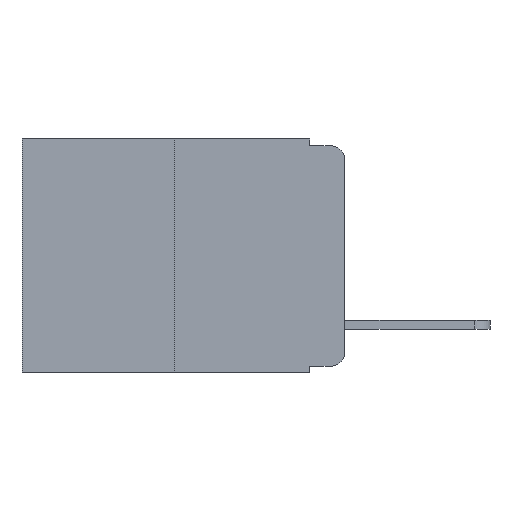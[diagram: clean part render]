
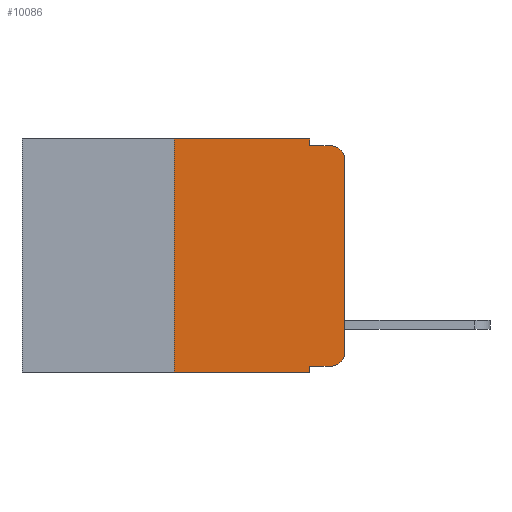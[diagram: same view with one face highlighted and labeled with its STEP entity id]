
A CAD part, left-side view. The second image highlights one B-rep face of the part: STEP entity #10086.
In plain terms, the highlighted planar face has unit normal (-1, 0, 0).
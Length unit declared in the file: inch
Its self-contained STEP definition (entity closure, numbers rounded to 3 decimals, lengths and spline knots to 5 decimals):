
#522 = VERTEX_POINT ( 'NONE', #17856 ) ;
#635 = EDGE_LOOP ( 'NONE', ( #8766, #15055, #14808, #16039, #1866, #13015, #6742, #17169, #10943, #3897 ) ) ;
#1286 = VERTEX_POINT ( 'NONE', #6475 ) ;
#1456 = CARTESIAN_POINT ( 'NONE',  ( 0., 0.473, 0. ) ) ;
#1482 = VECTOR ( 'NONE', #19501, 39.37008 ) ;
#1515 = VERTEX_POINT ( 'NONE', #21217 ) ;
#1670 = VERTEX_POINT ( 'NONE', #19282 ) ;
#1773 = VERTEX_POINT ( 'NONE', #13369 ) ;
#1866 = ORIENTED_EDGE ( 'NONE', *, *, #22059, .F. ) ;
#2009 = CARTESIAN_POINT ( 'NONE',  ( 0., 0.051, 0. ) ) ;
#2374 = DIRECTION ( 'NONE',  ( 0., -1., 0. ) ) ;
#2985 = DIRECTION ( 'NONE',  ( 1., 0., 0. ) ) ;
#3339 = LINE ( 'NONE', #13396, #12637 ) ;
#3429 = CARTESIAN_POINT ( 'NONE',  ( 0., 0.25, 0. ) ) ;
#3896 = CARTESIAN_POINT ( 'NONE',  ( 0., 0.02, -0.03 ) ) ;
#3897 = ORIENTED_EDGE ( 'NONE', *, *, #13821, .T. ) ;
#4134 = CARTESIAN_POINT ( 'NONE',  ( 0., 0., 0. ) ) ;
#4506 = LINE ( 'NONE', #16288, #18839 ) ;
#4828 = DIRECTION ( 'NONE',  ( -1., 0., 0. ) ) ;
#5191 = FACE_OUTER_BOUND ( 'NONE', #635, .T. ) ;
#5211 = AXIS2_PLACEMENT_3D ( 'NONE', #15558, #4828, #17143 ) ;
#5690 = DIRECTION ( 'NONE',  ( 0., 0., -1. ) ) ;
#5777 = DIRECTION ( 'NONE',  ( 0., 0., -1. ) ) ;
#5843 = VERTEX_POINT ( 'NONE', #11547 ) ;
#6475 = CARTESIAN_POINT ( 'NONE',  ( 0., 0., -0.313 ) ) ;
#6742 = ORIENTED_EDGE ( 'NONE', *, *, #8950, .T. ) ;
#7305 = VECTOR ( 'NONE', #17511, 39.37008 ) ;
#8766 = ORIENTED_EDGE ( 'NONE', *, *, #12024, .T. ) ;
#8950 = EDGE_CURVE ( 'NONE', #10830, #11506, #15998, .T. ) ;
#9763 = CARTESIAN_POINT ( 'NONE',  ( 0., 0.051, 0. ) ) ;
#9830 = LINE ( 'NONE', #10419, #22163 ) ;
#10086 = ADVANCED_FACE ( 'NONE', ( #5191 ), #12290, .F. ) ;
#10419 = CARTESIAN_POINT ( 'NONE',  ( 0., 0.051, -0.01 ) ) ;
#10495 = CARTESIAN_POINT ( 'NONE',  ( 0., 0.473, 0. ) ) ;
#10830 = VERTEX_POINT ( 'NONE', #17110 ) ;
#10943 = ORIENTED_EDGE ( 'NONE', *, *, #11575, .T. ) ;
#10970 = VECTOR ( 'NONE', #21065, 39.37008 ) ;
#11149 = CIRCLE ( 'NONE', #5211, 0.02 ) ;
#11404 = EDGE_CURVE ( 'NONE', #10830, #1773, #14459, .T. ) ;
#11461 = CARTESIAN_POINT ( 'NONE',  ( 0., 0.051, -0.343 ) ) ;
#11506 = VERTEX_POINT ( 'NONE', #11461 ) ;
#11518 = EDGE_CURVE ( 'NONE', #1515, #11506, #22417, .T. ) ;
#11547 = CARTESIAN_POINT ( 'NONE',  ( 0., 0.051, -0.01 ) ) ;
#11575 = EDGE_CURVE ( 'NONE', #1515, #12479, #3339, .T. ) ;
#11635 = CARTESIAN_POINT ( 'NONE',  ( 0., 0.02, -0.333 ) ) ;
#11679 = EDGE_CURVE ( 'NONE', #5843, #522, #9830, .T. ) ;
#11948 = EDGE_CURVE ( 'NONE', #18421, #5843, #4506, .T. ) ;
#11957 = EDGE_CURVE ( 'NONE', #1670, #522, #13150, .T. ) ;
#12024 = EDGE_CURVE ( 'NONE', #1286, #1670, #19547, .T. ) ;
#12216 = DIRECTION ( 'NONE',  ( 0., -1., 0. ) ) ;
#12290 = PLANE ( 'NONE',  #21324 ) ;
#12479 = VERTEX_POINT ( 'NONE', #11635 ) ;
#12637 = VECTOR ( 'NONE', #2374, 39.37008 ) ;
#13015 = ORIENTED_EDGE ( 'NONE', *, *, #11404, .F. ) ;
#13150 = CIRCLE ( 'NONE', #21230, 0.02 ) ;
#13369 = CARTESIAN_POINT ( 'NONE',  ( 0., 0.25, 0. ) ) ;
#13396 = CARTESIAN_POINT ( 'NONE',  ( 0., 0.051, -0.333 ) ) ;
#13821 = EDGE_CURVE ( 'NONE', #12479, #1286, #11149, .T. ) ;
#14459 = LINE ( 'NONE', #3429, #18149 ) ;
#14808 = ORIENTED_EDGE ( 'NONE', *, *, #11679, .F. ) ;
#15055 = ORIENTED_EDGE ( 'NONE', *, *, #11957, .T. ) ;
#15558 = CARTESIAN_POINT ( 'NONE',  ( 0., 0.02, -0.313 ) ) ;
#15622 = DIRECTION ( 'NONE',  ( 0., 0., -1. ) ) ;
#15998 = LINE ( 'NONE', #17973, #1482 ) ;
#16039 = ORIENTED_EDGE ( 'NONE', *, *, #11948, .F. ) ;
#16288 = CARTESIAN_POINT ( 'NONE',  ( 0., 0.051, 0. ) ) ;
#16359 = DIRECTION ( 'NONE',  ( -1., 0., 0. ) ) ;
#17110 = CARTESIAN_POINT ( 'NONE',  ( 0., 0.25, -0.343 ) ) ;
#17143 = DIRECTION ( 'NONE',  ( 0., 0., -1. ) ) ;
#17169 = ORIENTED_EDGE ( 'NONE', *, *, #11518, .F. ) ;
#17511 = DIRECTION ( 'NONE',  ( 0., -1., 0. ) ) ;
#17856 = CARTESIAN_POINT ( 'NONE',  ( 0., 0.02, -0.01 ) ) ;
#17973 = CARTESIAN_POINT ( 'NONE',  ( 0., 0.473, -0.343 ) ) ;
#18149 = VECTOR ( 'NONE', #19057, 39.37008 ) ;
#18373 = VECTOR ( 'NONE', #21030, 39.37008 ) ;
#18421 = VERTEX_POINT ( 'NONE', #9763 ) ;
#18839 = VECTOR ( 'NONE', #5690, 39.37008 ) ;
#19057 = DIRECTION ( 'NONE',  ( 0., 0., 1. ) ) ;
#19282 = CARTESIAN_POINT ( 'NONE',  ( 0., 0., -0.03 ) ) ;
#19501 = DIRECTION ( 'NONE',  ( 0., -1., 0. ) ) ;
#19547 = LINE ( 'NONE', #4134, #10970 ) ;
#20592 = LINE ( 'NONE', #1456, #7305 ) ;
#21030 = DIRECTION ( 'NONE',  ( 0., 0., -1. ) ) ;
#21065 = DIRECTION ( 'NONE',  ( 0., 0., 1. ) ) ;
#21217 = CARTESIAN_POINT ( 'NONE',  ( 0., 0.051, -0.333 ) ) ;
#21230 = AXIS2_PLACEMENT_3D ( 'NONE', #3896, #16359, #5777 ) ;
#21324 = AXIS2_PLACEMENT_3D ( 'NONE', #10495, #2985, #15622 ) ;
#22059 = EDGE_CURVE ( 'NONE', #1773, #18421, #20592, .T. ) ;
#22163 = VECTOR ( 'NONE', #12216, 39.37008 ) ;
#22417 = LINE ( 'NONE', #2009, #18373 ) ;
